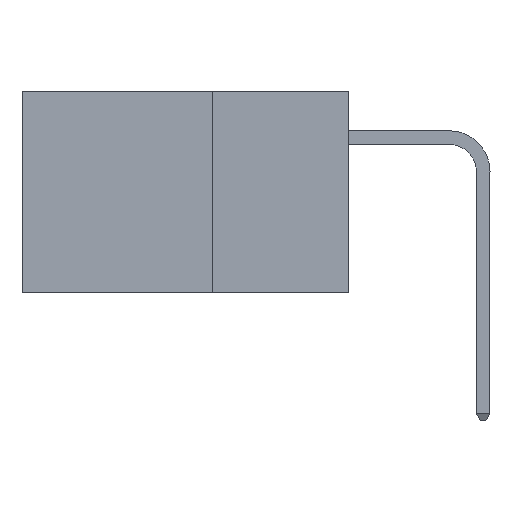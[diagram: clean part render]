
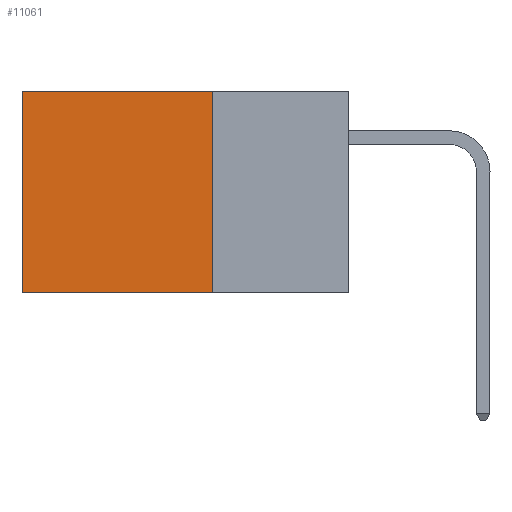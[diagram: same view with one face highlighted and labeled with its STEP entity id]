
A CAD part, left-side view. The second image highlights one B-rep face of the part: STEP entity #11061.
In plain terms, the highlighted planar face has unit normal (-1, 0, 0).
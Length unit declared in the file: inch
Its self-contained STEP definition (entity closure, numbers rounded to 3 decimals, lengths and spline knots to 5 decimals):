
#2001 = LINE ( 'NONE', #14826, #31695 ) ;
#3586 = DIRECTION ( 'NONE',  ( 0., 0., -1. ) ) ;
#4701 = CARTESIAN_POINT ( 'NONE',  ( 0.2875, 0.25, -0.37 ) ) ;
#5709 = EDGE_CURVE ( 'NONE', #30549, #23102, #33888, .T. ) ;
#6151 = DIRECTION ( 'NONE',  ( 0., 0., -1. ) ) ;
#6921 = DIRECTION ( 'NONE',  ( 0., 1., 0. ) ) ;
#7149 = VERTEX_POINT ( 'NONE', #4701 ) ;
#9019 = CARTESIAN_POINT ( 'NONE',  ( 0.2875, 0.25, 0. ) ) ;
#9121 = VECTOR ( 'NONE', #6151, 39.37008 ) ;
#9182 = VECTOR ( 'NONE', #6921, 39.37008 ) ;
#9488 = ORIENTED_EDGE ( 'NONE', *, *, #14267, .F. ) ;
#10848 = CARTESIAN_POINT ( 'NONE',  ( 0.2875, 0.6, -0.37 ) ) ;
#11061 = ADVANCED_FACE ( 'NONE', ( #16490 ), #12143, .F. ) ;
#11907 = DIRECTION ( 'NONE',  ( 0., 0., -1. ) ) ;
#12143 = PLANE ( 'NONE',  #18112 ) ;
#12308 = EDGE_CURVE ( 'NONE', #7149, #23102, #2001, .T. ) ;
#14028 = ORIENTED_EDGE ( 'NONE', *, *, #5709, .T. ) ;
#14267 = EDGE_CURVE ( 'NONE', #26052, #7149, #30697, .T. ) ;
#14826 = CARTESIAN_POINT ( 'NONE',  ( 0.2875, 0.25, -0.37 ) ) ;
#15044 = CARTESIAN_POINT ( 'NONE',  ( 0.2875, 0.25, 0. ) ) ;
#15378 = VECTOR ( 'NONE', #11907, 39.37008 ) ;
#16490 = FACE_OUTER_BOUND ( 'NONE', #31373, .T. ) ;
#17735 = DIRECTION ( 'NONE',  ( 0., 1., 0. ) ) ;
#18112 = AXIS2_PLACEMENT_3D ( 'NONE', #15044, #20822, #3586 ) ;
#20474 = ORIENTED_EDGE ( 'NONE', *, *, #12308, .F. ) ;
#20822 = DIRECTION ( 'NONE',  ( 1., 0., 0. ) ) ;
#22096 = CARTESIAN_POINT ( 'NONE',  ( 0.2875, 0.6, 0. ) ) ;
#23102 = VERTEX_POINT ( 'NONE', #10848 ) ;
#24505 = LINE ( 'NONE', #32769, #9182 ) ;
#26052 = VERTEX_POINT ( 'NONE', #28206 ) ;
#28206 = CARTESIAN_POINT ( 'NONE',  ( 0.2875, 0.25, 0. ) ) ;
#29057 = EDGE_CURVE ( 'NONE', #26052, #30549, #24505, .T. ) ;
#30549 = VERTEX_POINT ( 'NONE', #22096 ) ;
#30697 = LINE ( 'NONE', #9019, #15378 ) ;
#31373 = EDGE_LOOP ( 'NONE', ( #14028, #20474, #9488, #36799 ) ) ;
#31695 = VECTOR ( 'NONE', #17735, 39.37008 ) ;
#32122 = CARTESIAN_POINT ( 'NONE',  ( 0.2875, 0.6, 0. ) ) ;
#32769 = CARTESIAN_POINT ( 'NONE',  ( 0.2875, 0.25, 0. ) ) ;
#33888 = LINE ( 'NONE', #32122, #9121 ) ;
#36799 = ORIENTED_EDGE ( 'NONE', *, *, #29057, .T. ) ;
